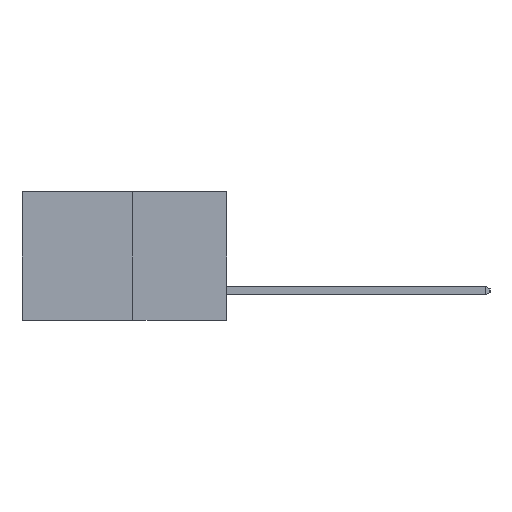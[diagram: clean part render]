
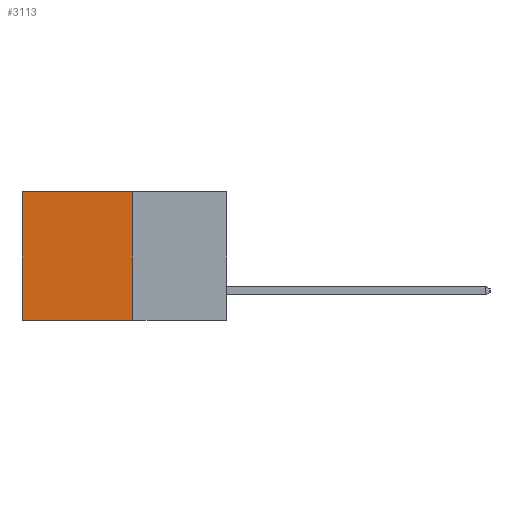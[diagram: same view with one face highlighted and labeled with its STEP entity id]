
A CAD part, left-side view. The second image highlights one B-rep face of the part: STEP entity #3113.
In plain terms, the highlighted planar face has unit normal (-1, 0, 0).
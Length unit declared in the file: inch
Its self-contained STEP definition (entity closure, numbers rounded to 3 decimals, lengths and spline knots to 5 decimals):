
#576 = LINE ( 'NONE', #12202, #2947 ) ;
#581 = VERTEX_POINT ( 'NONE', #1221 ) ;
#996 = CARTESIAN_POINT ( 'NONE',  ( 0.277, 0.59, -0.37 ) ) ;
#1042 = VECTOR ( 'NONE', #4771, 39.37008 ) ;
#1221 = CARTESIAN_POINT ( 'NONE',  ( 0.277, 0.27, 0. ) ) ;
#1350 = LINE ( 'NONE', #10351, #1042 ) ;
#1408 = ORIENTED_EDGE ( 'NONE', *, *, #3282, .T. ) ;
#1746 = ORIENTED_EDGE ( 'NONE', *, *, #3351, .T. ) ;
#2490 = FACE_OUTER_BOUND ( 'NONE', #5133, .T. ) ;
#2651 = LINE ( 'NONE', #11648, #5220 ) ;
#2947 = VECTOR ( 'NONE', #12085, 39.37008 ) ;
#3113 = ADVANCED_FACE ( 'NONE', ( #2490 ), #3616, .F. ) ;
#3282 = EDGE_CURVE ( 'NONE', #11245, #4472, #576, .T. ) ;
#3351 = EDGE_CURVE ( 'NONE', #581, #11245, #2651, .T. ) ;
#3369 = DIRECTION ( 'NONE',  ( 0., 0., -1. ) ) ;
#3372 = VERTEX_POINT ( 'NONE', #11528 ) ;
#3552 = DIRECTION ( 'NONE',  ( 1., 0., 0. ) ) ;
#3616 = PLANE ( 'NONE',  #8239 ) ;
#3723 = CARTESIAN_POINT ( 'NONE',  ( 0.277, 0.27, -0.37 ) ) ;
#4007 = ORIENTED_EDGE ( 'NONE', *, *, #5239, .F. ) ;
#4406 = VECTOR ( 'NONE', #8696, 39.37008 ) ;
#4472 = VERTEX_POINT ( 'NONE', #996 ) ;
#4771 = DIRECTION ( 'NONE',  ( 0., 1., 0. ) ) ;
#5133 = EDGE_LOOP ( 'NONE', ( #1408, #4007, #11461, #1746 ) ) ;
#5220 = VECTOR ( 'NONE', #11705, 39.37008 ) ;
#5239 = EDGE_CURVE ( 'NONE', #3372, #4472, #1350, .T. ) ;
#5403 = EDGE_CURVE ( 'NONE', #581, #3372, #11831, .T. ) ;
#7762 = CARTESIAN_POINT ( 'NONE',  ( 0.277, 0.27, -0.37 ) ) ;
#8239 = AXIS2_PLACEMENT_3D ( 'NONE', #3723, #3552, #3369 ) ;
#8696 = DIRECTION ( 'NONE',  ( 0., 0., -1. ) ) ;
#8742 = CARTESIAN_POINT ( 'NONE',  ( 0.277, 0.59, 0. ) ) ;
#10351 = CARTESIAN_POINT ( 'NONE',  ( 0.277, 0.27, -0.37 ) ) ;
#11245 = VERTEX_POINT ( 'NONE', #8742 ) ;
#11461 = ORIENTED_EDGE ( 'NONE', *, *, #5403, .F. ) ;
#11528 = CARTESIAN_POINT ( 'NONE',  ( 0.277, 0.27, -0.37 ) ) ;
#11648 = CARTESIAN_POINT ( 'NONE',  ( 0.277, 0.27, 0. ) ) ;
#11705 = DIRECTION ( 'NONE',  ( 0., 1., 0. ) ) ;
#11831 = LINE ( 'NONE', #7762, #4406 ) ;
#12085 = DIRECTION ( 'NONE',  ( 0., 0., -1. ) ) ;
#12202 = CARTESIAN_POINT ( 'NONE',  ( 0.277, 0.59, -0.37 ) ) ;
